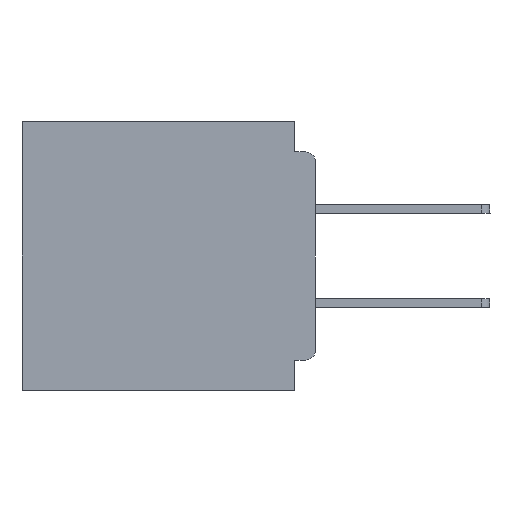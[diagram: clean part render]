
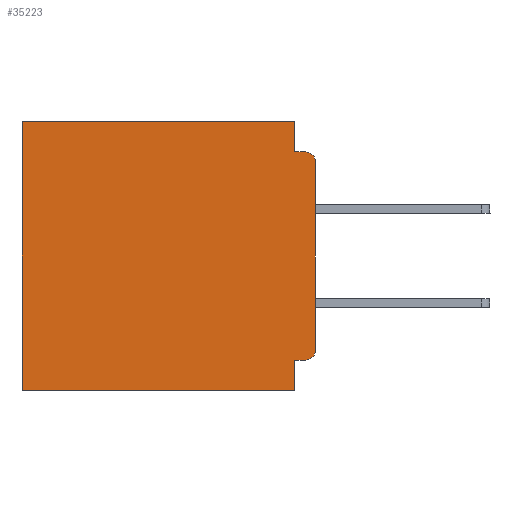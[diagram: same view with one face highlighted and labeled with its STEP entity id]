
A CAD part, left-side view. The second image highlights one B-rep face of the part: STEP entity #35223.
In plain terms, the highlighted planar face has unit normal (-1, 0, 0).
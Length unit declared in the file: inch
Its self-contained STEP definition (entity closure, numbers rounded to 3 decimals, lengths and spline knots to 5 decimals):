
#563 = CARTESIAN_POINT ( 'NONE',  ( 0.3, 0.015, -0.045 ) ) ;
#701 = DIRECTION ( 'NONE',  ( 0., 0., -1. ) ) ;
#2015 = CARTESIAN_POINT ( 'NONE',  ( 0.3, 0., -0.355 ) ) ;
#2686 = DIRECTION ( 'NONE',  ( 0., 0., -1. ) ) ;
#2891 = ORIENTED_EDGE ( 'NONE', *, *, #6652, .T. ) ;
#3344 = CARTESIAN_POINT ( 'NONE',  ( 0.3, 0.031, -0.355 ) ) ;
#3772 = EDGE_CURVE ( 'NONE', #50094, #4245, #37390, .T. ) ;
#4245 = VERTEX_POINT ( 'NONE', #12147 ) ;
#4599 = VERTEX_POINT ( 'NONE', #22949 ) ;
#6652 = EDGE_CURVE ( 'NONE', #11160, #18006, #34573, .T. ) ;
#7247 = ORIENTED_EDGE ( 'NONE', *, *, #46192, .T. ) ;
#7573 = CARTESIAN_POINT ( 'NONE',  ( 0.3, 0.437, 0. ) ) ;
#8360 = VECTOR ( 'NONE', #701, 39.37008 ) ;
#8851 = ORIENTED_EDGE ( 'NONE', *, *, #3772, .F. ) ;
#8953 = CARTESIAN_POINT ( 'NONE',  ( 0.3, 0., -0.4 ) ) ;
#10193 = CIRCLE ( 'NONE', #49854, 0.015 ) ;
#11160 = VERTEX_POINT ( 'NONE', #53330 ) ;
#11310 = EDGE_CURVE ( 'NONE', #4599, #34667, #19829, .T. ) ;
#11593 = VERTEX_POINT ( 'NONE', #7573 ) ;
#12147 = CARTESIAN_POINT ( 'NONE',  ( 0.3, 0.031, -0.4 ) ) ;
#12942 = DIRECTION ( 'NONE',  ( -1., 0., 0. ) ) ;
#13950 = VERTEX_POINT ( 'NONE', #56948 ) ;
#14904 = ORIENTED_EDGE ( 'NONE', *, *, #43213, .F. ) ;
#15769 = CARTESIAN_POINT ( 'NONE',  ( 0.3, 0.437, -0.4 ) ) ;
#16588 = VECTOR ( 'NONE', #39391, 39.37008 ) ;
#17914 = LINE ( 'NONE', #27476, #29839 ) ;
#18006 = VERTEX_POINT ( 'NONE', #32975 ) ;
#18267 = VECTOR ( 'NONE', #52797, 39.37008 ) ;
#19829 = LINE ( 'NONE', #24140, #16588 ) ;
#19856 = ORIENTED_EDGE ( 'NONE', *, *, #11310, .F. ) ;
#20535 = CARTESIAN_POINT ( 'NONE',  ( 0.3, 0.015, -0.34 ) ) ;
#20614 = AXIS2_PLACEMENT_3D ( 'NONE', #20535, #55945, #25646 ) ;
#20895 = LINE ( 'NONE', #8953, #47799 ) ;
#22085 = EDGE_CURVE ( 'NONE', #4245, #49127, #17914, .T. ) ;
#22742 = CARTESIAN_POINT ( 'NONE',  ( 0.3, 0., 0. ) ) ;
#22949 = CARTESIAN_POINT ( 'NONE',  ( 0.3, 0.031, -0.045 ) ) ;
#23527 = LINE ( 'NONE', #15769, #8360 ) ;
#23621 = LINE ( 'NONE', #22742, #48903 ) ;
#24140 = CARTESIAN_POINT ( 'NONE',  ( 0.3, 0., -0.045 ) ) ;
#25039 = ORIENTED_EDGE ( 'NONE', *, *, #41638, .T. ) ;
#25646 = DIRECTION ( 'NONE',  ( 0., 0., -1. ) ) ;
#27476 = CARTESIAN_POINT ( 'NONE',  ( 0.3, 0., -0.4 ) ) ;
#29131 = ORIENTED_EDGE ( 'NONE', *, *, #55997, .F. ) ;
#29839 = VECTOR ( 'NONE', #52681, 39.37008 ) ;
#31749 = LINE ( 'NONE', #2015, #18267 ) ;
#32928 = ORIENTED_EDGE ( 'NONE', *, *, #22085, .F. ) ;
#32975 = CARTESIAN_POINT ( 'NONE',  ( 0.3, 0., -0.34 ) ) ;
#33068 = DIRECTION ( 'NONE',  ( 1., 0., 0. ) ) ;
#33937 = LINE ( 'NONE', #47014, #59285 ) ;
#34573 = CIRCLE ( 'NONE', #20614, 0.015 ) ;
#34667 = VERTEX_POINT ( 'NONE', #563 ) ;
#34896 = EDGE_LOOP ( 'NONE', ( #14904, #46853, #19856, #29131, #7247, #25039, #32928, #8851, #41530, #2891 ) ) ;
#35158 = EDGE_CURVE ( 'NONE', #11160, #50094, #31749, .T. ) ;
#35223 = ADVANCED_FACE ( 'NONE', ( #45225 ), #63362, .F. ) ;
#37390 = LINE ( 'NONE', #40048, #62656 ) ;
#39391 = DIRECTION ( 'NONE',  ( 0., -1., 0. ) ) ;
#40048 = CARTESIAN_POINT ( 'NONE',  ( 0.3, 0.031, -0.4 ) ) ;
#41530 = ORIENTED_EDGE ( 'NONE', *, *, #35158, .F. ) ;
#41638 = EDGE_CURVE ( 'NONE', #11593, #49127, #23527, .T. ) ;
#43213 = EDGE_CURVE ( 'NONE', #43394, #18006, #20895, .T. ) ;
#43352 = CARTESIAN_POINT ( 'NONE',  ( 0.3, 0.015, -0.06 ) ) ;
#43394 = VERTEX_POINT ( 'NONE', #55928 ) ;
#44310 = CARTESIAN_POINT ( 'NONE',  ( 0.3, 0.437, -0.4 ) ) ;
#44442 = DIRECTION ( 'NONE',  ( 0., 0., -1. ) ) ;
#45225 = FACE_OUTER_BOUND ( 'NONE', #34896, .T. ) ;
#46192 = EDGE_CURVE ( 'NONE', #13950, #11593, #23621, .T. ) ;
#46853 = ORIENTED_EDGE ( 'NONE', *, *, #55518, .T. ) ;
#47014 = CARTESIAN_POINT ( 'NONE',  ( 0.3, 0.031, 0. ) ) ;
#47799 = VECTOR ( 'NONE', #44442, 39.37008 ) ;
#48130 = CARTESIAN_POINT ( 'NONE',  ( 0.3, 0., -0.4 ) ) ;
#48408 = DIRECTION ( 'NONE',  ( 0., 0., -1. ) ) ;
#48903 = VECTOR ( 'NONE', #63178, 39.37008 ) ;
#49127 = VERTEX_POINT ( 'NONE', #44310 ) ;
#49854 = AXIS2_PLACEMENT_3D ( 'NONE', #43352, #12942, #48408 ) ;
#50094 = VERTEX_POINT ( 'NONE', #3344 ) ;
#52121 = DIRECTION ( 'NONE',  ( 0., 0., -1. ) ) ;
#52681 = DIRECTION ( 'NONE',  ( 0., 1., 0. ) ) ;
#52797 = DIRECTION ( 'NONE',  ( 0., 1., 0. ) ) ;
#52985 = AXIS2_PLACEMENT_3D ( 'NONE', #48130, #33068, #2686 ) ;
#53330 = CARTESIAN_POINT ( 'NONE',  ( 0.3, 0.015, -0.355 ) ) ;
#53615 = DIRECTION ( 'NONE',  ( 0., 0., -1. ) ) ;
#55518 = EDGE_CURVE ( 'NONE', #43394, #34667, #10193, .T. ) ;
#55928 = CARTESIAN_POINT ( 'NONE',  ( 0.3, 0., -0.06 ) ) ;
#55945 = DIRECTION ( 'NONE',  ( -1., 0., 0. ) ) ;
#55997 = EDGE_CURVE ( 'NONE', #13950, #4599, #33937, .T. ) ;
#56948 = CARTESIAN_POINT ( 'NONE',  ( 0.3, 0.031, 0. ) ) ;
#59285 = VECTOR ( 'NONE', #52121, 39.37008 ) ;
#62656 = VECTOR ( 'NONE', #53615, 39.37008 ) ;
#63178 = DIRECTION ( 'NONE',  ( 0., 1., 0. ) ) ;
#63362 = PLANE ( 'NONE',  #52985 ) ;
